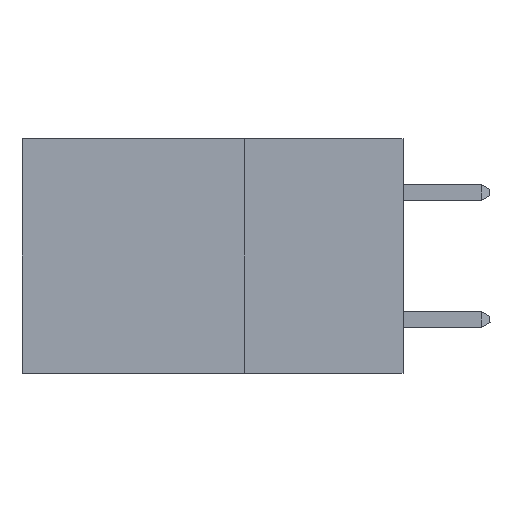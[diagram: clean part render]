
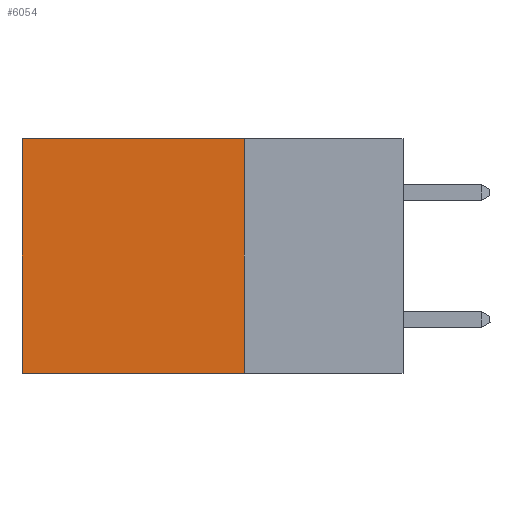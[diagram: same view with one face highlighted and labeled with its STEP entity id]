
A CAD part, left-side view. The second image highlights one B-rep face of the part: STEP entity #6054.
In plain terms, the highlighted planar face has unit normal (-1, 0, 0).
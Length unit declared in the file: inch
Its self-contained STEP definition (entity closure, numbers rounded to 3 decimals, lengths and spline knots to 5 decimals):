
#198 = CARTESIAN_POINT ( 'NONE',  ( 0.2875, 0.25, 0. ) ) ;
#762 = EDGE_CURVE ( 'NONE', #7546, #5463, #7883, .T. ) ;
#1301 = ORIENTED_EDGE ( 'NONE', *, *, #11754, .F. ) ;
#1388 = EDGE_CURVE ( 'NONE', #5463, #11174, #16460, .T. ) ;
#1766 = DIRECTION ( 'NONE',  ( 1., 0., 0. ) ) ;
#2943 = VECTOR ( 'NONE', #12602, 39.37008 ) ;
#3142 = DIRECTION ( 'NONE',  ( 0., 0., -1. ) ) ;
#4237 = EDGE_CURVE ( 'NONE', #10633, #11174, #5016, .T. ) ;
#4666 = CARTESIAN_POINT ( 'NONE',  ( 0.2875, 0.25, 0. ) ) ;
#4863 = FACE_OUTER_BOUND ( 'NONE', #17986, .T. ) ;
#5016 = LINE ( 'NONE', #10936, #5791 ) ;
#5463 = VERTEX_POINT ( 'NONE', #17445 ) ;
#5646 = DIRECTION ( 'NONE',  ( 0., 0., -1. ) ) ;
#5791 = VECTOR ( 'NONE', #9528, 39.37008 ) ;
#6054 = ADVANCED_FACE ( 'NONE', ( #4863 ), #18172, .F. ) ;
#7546 = VERTEX_POINT ( 'NONE', #15357 ) ;
#7883 = LINE ( 'NONE', #198, #2943 ) ;
#9528 = DIRECTION ( 'NONE',  ( 0., 1., 0. ) ) ;
#10344 = VECTOR ( 'NONE', #5646, 39.37008 ) ;
#10633 = VERTEX_POINT ( 'NONE', #13431 ) ;
#10936 = CARTESIAN_POINT ( 'NONE',  ( 0.2875, 0.25, -0.37 ) ) ;
#11174 = VERTEX_POINT ( 'NONE', #19479 ) ;
#11203 = ORIENTED_EDGE ( 'NONE', *, *, #1388, .T. ) ;
#11525 = ORIENTED_EDGE ( 'NONE', *, *, #4237, .F. ) ;
#11754 = EDGE_CURVE ( 'NONE', #7546, #10633, #18431, .T. ) ;
#12602 = DIRECTION ( 'NONE',  ( 0., 1., 0. ) ) ;
#13431 = CARTESIAN_POINT ( 'NONE',  ( 0.2875, 0.25, -0.37 ) ) ;
#15070 = DIRECTION ( 'NONE',  ( 0., 0., -1. ) ) ;
#15357 = CARTESIAN_POINT ( 'NONE',  ( 0.2875, 0.25, 0. ) ) ;
#16170 = CARTESIAN_POINT ( 'NONE',  ( 0.2875, 0.6, 0. ) ) ;
#16460 = LINE ( 'NONE', #16170, #10344 ) ;
#16515 = VECTOR ( 'NONE', #3142, 39.37008 ) ;
#16729 = AXIS2_PLACEMENT_3D ( 'NONE', #4666, #1766, #15070 ) ;
#16845 = CARTESIAN_POINT ( 'NONE',  ( 0.2875, 0.25, 0. ) ) ;
#17445 = CARTESIAN_POINT ( 'NONE',  ( 0.2875, 0.6, 0. ) ) ;
#17986 = EDGE_LOOP ( 'NONE', ( #11203, #11525, #1301, #18400 ) ) ;
#18172 = PLANE ( 'NONE',  #16729 ) ;
#18400 = ORIENTED_EDGE ( 'NONE', *, *, #762, .T. ) ;
#18431 = LINE ( 'NONE', #16845, #16515 ) ;
#19479 = CARTESIAN_POINT ( 'NONE',  ( 0.2875, 0.6, -0.37 ) ) ;
